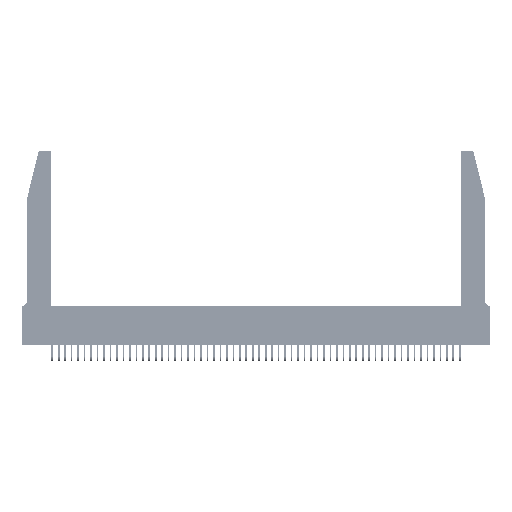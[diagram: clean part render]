
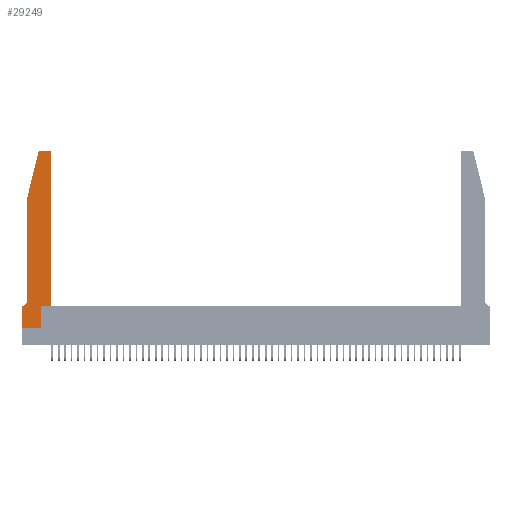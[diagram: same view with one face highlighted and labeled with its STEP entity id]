
A CAD part, top view. The second image highlights one B-rep face of the part: STEP entity #29249.
In plain terms, the highlighted planar face has unit normal (0, 0, 1).
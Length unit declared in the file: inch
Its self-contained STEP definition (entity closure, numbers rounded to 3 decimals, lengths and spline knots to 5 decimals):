
#13 = VERTEX_POINT ( 'NONE', #43269 ) ;
#477 = ORIENTED_EDGE ( 'NONE', *, *, #41857, .T. ) ;
#1962 = VERTEX_POINT ( 'NONE', #44601 ) ;
#2423 = CARTESIAN_POINT ( 'NONE',  ( 0.25487, 2.72718, 0.37 ) ) ;
#2749 = DIRECTION ( 'NONE',  ( 0., 0., 1. ) ) ;
#3754 = EDGE_CURVE ( 'NONE', #13, #3945, #23463, .T. ) ;
#3945 = VERTEX_POINT ( 'NONE', #36040 ) ;
#4239 = LINE ( 'NONE', #30623, #26267 ) ;
#4518 = ORIENTED_EDGE ( 'NONE', *, *, #8782, .T. ) ;
#4931 = CARTESIAN_POINT ( 'NONE',  ( 0.0755, 2., 0.37 ) ) ;
#5885 = EDGE_CURVE ( 'NONE', #13325, #50825, #21510, .T. ) ;
#7502 = ORIENTED_EDGE ( 'NONE', *, *, #5885, .T. ) ;
#7620 = EDGE_CURVE ( 'NONE', #1962, #18507, #21358, .T. ) ;
#8782 = EDGE_CURVE ( 'NONE', #14826, #40750, #47160, .T. ) ;
#9160 = CARTESIAN_POINT ( 'NONE',  ( 0.0055, 0.42, 0.37 ) ) ;
#9921 = VERTEX_POINT ( 'NONE', #24032 ) ;
#10265 = VECTOR ( 'NONE', #10416, 39.37008 ) ;
#10416 = DIRECTION ( 'NONE',  ( -1., 0., 0. ) ) ;
#10611 = DIRECTION ( 'NONE',  ( 0., -1., 0. ) ) ;
#10787 = AXIS2_PLACEMENT_3D ( 'NONE', #30996, #2749, #43507 ) ;
#11933 = PLANE ( 'NONE',  #40035 ) ;
#13325 = VERTEX_POINT ( 'NONE', #15258 ) ;
#13695 = DIRECTION ( 'NONE',  ( -1., 0., 0. ) ) ;
#14826 = VERTEX_POINT ( 'NONE', #49517 ) ;
#14926 = EDGE_CURVE ( 'NONE', #3945, #13325, #50405, .T. ) ;
#15258 = CARTESIAN_POINT ( 'NONE',  ( 0.284, 2.75, 0.37 ) ) ;
#15772 = ORIENTED_EDGE ( 'NONE', *, *, #7620, .T. ) ;
#16078 = CARTESIAN_POINT ( 'NONE',  ( 0., 0.35, 0.37 ) ) ;
#16419 = DIRECTION ( 'NONE',  ( 1., 0., 0. ) ) ;
#16601 = CARTESIAN_POINT ( 'NONE',  ( 0., 0.35, 0.37 ) ) ;
#17073 = VERTEX_POINT ( 'NONE', #16078 ) ;
#17509 = CARTESIAN_POINT ( 'NONE',  ( 0.284, 2.72, 0.37 ) ) ;
#17598 = VERTEX_POINT ( 'NONE', #18398 ) ;
#17709 = DIRECTION ( 'NONE',  ( 1., 0., 0. ) ) ;
#17830 = DIRECTION ( 'NONE',  ( 0., 0., -1. ) ) ;
#18398 = CARTESIAN_POINT ( 'NONE',  ( 0.2865, 0., 0.37 ) ) ;
#18467 = AXIS2_PLACEMENT_3D ( 'NONE', #17509, #29643, #34149 ) ;
#18507 = VERTEX_POINT ( 'NONE', #27167 ) ;
#18549 = FACE_OUTER_BOUND ( 'NONE', #23459, .T. ) ;
#18936 = CARTESIAN_POINT ( 'NONE',  ( 0., 0., 0.37 ) ) ;
#20277 = CARTESIAN_POINT ( 'NONE',  ( 0.0755, 0.42, 0.37 ) ) ;
#20429 = VERTEX_POINT ( 'NONE', #39899 ) ;
#20885 = VECTOR ( 'NONE', #49157, 39.37008 ) ;
#21242 = VECTOR ( 'NONE', #29200, 39.37008 ) ;
#21290 = LINE ( 'NONE', #43153, #10265 ) ;
#21343 = CARTESIAN_POINT ( 'NONE',  ( 0.2865, 0.35, 0.37 ) ) ;
#21358 = LINE ( 'NONE', #46693, #44665 ) ;
#21510 = CIRCLE ( 'NONE', #18467, 0.03 ) ;
#22156 = VECTOR ( 'NONE', #26174, 39.37008 ) ;
#23459 = EDGE_LOOP ( 'NONE', ( #35019, #7502, #28416, #4518, #477, #45715, #32996, #33820, #34361, #15772, #36480, #26161 ) ) ;
#23463 = CIRCLE ( 'NONE', #10787, 0.03 ) ;
#24032 = CARTESIAN_POINT ( 'NONE',  ( 0., 0., 0.37 ) ) ;
#24340 = CARTESIAN_POINT ( 'NONE',  ( 0.4505, 0.35, 0.37 ) ) ;
#26161 = ORIENTED_EDGE ( 'NONE', *, *, #3754, .T. ) ;
#26174 = DIRECTION ( 'NONE',  ( 0., 1., 0. ) ) ;
#26267 = VECTOR ( 'NONE', #43670, 39.37008 ) ;
#26399 = EDGE_CURVE ( 'NONE', #17598, #1962, #33113, .T. ) ;
#26873 = AXIS2_PLACEMENT_3D ( 'NONE', #9160, #17830, #13695 ) ;
#27167 = CARTESIAN_POINT ( 'NONE',  ( 0.4505, 0.35, 0.37 ) ) ;
#27170 = EDGE_CURVE ( 'NONE', #50825, #14826, #48635, .T. ) ;
#27883 = VECTOR ( 'NONE', #43704, 39.37008 ) ;
#28416 = ORIENTED_EDGE ( 'NONE', *, *, #27170, .T. ) ;
#29026 = DIRECTION ( 'NONE',  ( -1., 0., 0. ) ) ;
#29200 = DIRECTION ( 'NONE',  ( 0., -1., 0. ) ) ;
#29249 = ADVANCED_FACE ( 'NONE', ( #18549 ), #11933, .T. ) ;
#29643 = DIRECTION ( 'NONE',  ( 0., 0., 1. ) ) ;
#29745 = CARTESIAN_POINT ( 'NONE',  ( 0.2605, 2.75, 0.37 ) ) ;
#30623 = CARTESIAN_POINT ( 'NONE',  ( 0., 0., 0.37 ) ) ;
#30996 = CARTESIAN_POINT ( 'NONE',  ( 0.4205, 2.72, 0.37 ) ) ;
#32444 = EDGE_CURVE ( 'NONE', #18507, #13, #40259, .T. ) ;
#32996 = ORIENTED_EDGE ( 'NONE', *, *, #42013, .T. ) ;
#33113 = LINE ( 'NONE', #21343, #22156 ) ;
#33820 = ORIENTED_EDGE ( 'NONE', *, *, #36680, .T. ) ;
#34149 = DIRECTION ( 'NONE',  ( 1., 0., 0. ) ) ;
#34361 = ORIENTED_EDGE ( 'NONE', *, *, #26399, .T. ) ;
#35019 = ORIENTED_EDGE ( 'NONE', *, *, #14926, .T. ) ;
#36040 = CARTESIAN_POINT ( 'NONE',  ( 0.4205, 2.75, 0.37 ) ) ;
#36480 = ORIENTED_EDGE ( 'NONE', *, *, #32444, .T. ) ;
#36680 = EDGE_CURVE ( 'NONE', #9921, #17598, #4239, .T. ) ;
#37617 = LINE ( 'NONE', #18936, #40823 ) ;
#39899 = CARTESIAN_POINT ( 'NONE',  ( 0.0055, 0.35, 0.37 ) ) ;
#40035 = AXIS2_PLACEMENT_3D ( 'NONE', #16601, #49743, #16419 ) ;
#40259 = LINE ( 'NONE', #24340, #20885 ) ;
#40750 = VERTEX_POINT ( 'NONE', #20277 ) ;
#40823 = VECTOR ( 'NONE', #10611, 39.37008 ) ;
#41857 = EDGE_CURVE ( 'NONE', #40750, #20429, #44819, .T. ) ;
#42013 = EDGE_CURVE ( 'NONE', #17073, #9921, #37617, .T. ) ;
#43153 = CARTESIAN_POINT ( 'NONE',  ( 0.0755, 0.35, 0.37 ) ) ;
#43269 = CARTESIAN_POINT ( 'NONE',  ( 0.4505, 2.72, 0.37 ) ) ;
#43507 = DIRECTION ( 'NONE',  ( 1., 0., 0. ) ) ;
#43670 = DIRECTION ( 'NONE',  ( 1., 0., 0. ) ) ;
#43704 = DIRECTION ( 'NONE',  ( -0.239, -0.971, 0. ) ) ;
#44052 = CARTESIAN_POINT ( 'NONE',  ( 0.0755, 2., 0.37 ) ) ;
#44601 = CARTESIAN_POINT ( 'NONE',  ( 0.2865, 0.35, 0.37 ) ) ;
#44665 = VECTOR ( 'NONE', #17709, 39.37008 ) ;
#44819 = CIRCLE ( 'NONE', #26873, 0.07 ) ;
#45715 = ORIENTED_EDGE ( 'NONE', *, *, #51176, .T. ) ;
#46693 = CARTESIAN_POINT ( 'NONE',  ( 0.4505, 0.35, 0.37 ) ) ;
#47160 = LINE ( 'NONE', #4931, #21242 ) ;
#48635 = LINE ( 'NONE', #44052, #27883 ) ;
#49157 = DIRECTION ( 'NONE',  ( 0., 1., 0. ) ) ;
#49517 = CARTESIAN_POINT ( 'NONE',  ( 0.0755, 2., 0.37 ) ) ;
#49743 = DIRECTION ( 'NONE',  ( 0., 0., 1. ) ) ;
#50405 = LINE ( 'NONE', #29745, #51069 ) ;
#50825 = VERTEX_POINT ( 'NONE', #2423 ) ;
#51069 = VECTOR ( 'NONE', #29026, 39.37008 ) ;
#51176 = EDGE_CURVE ( 'NONE', #20429, #17073, #21290, .T. ) ;
